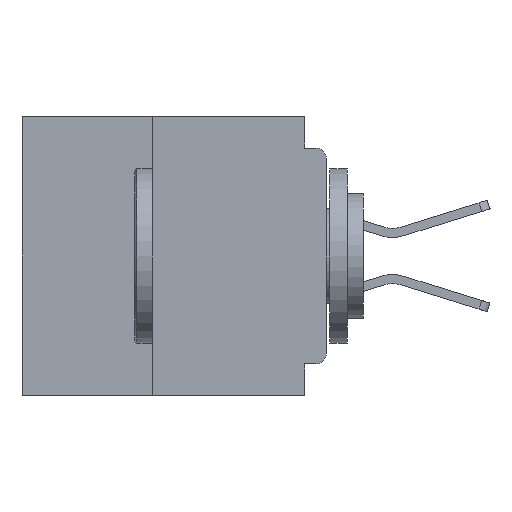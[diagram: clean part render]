
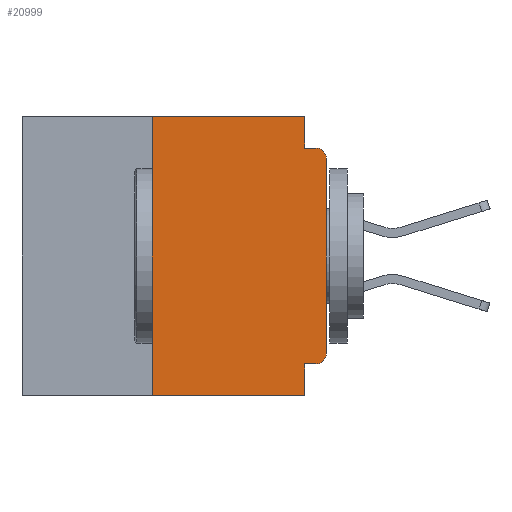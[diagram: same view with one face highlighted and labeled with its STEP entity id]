
A CAD part, left-side view. The second image highlights one B-rep face of the part: STEP entity #20999.
In plain terms, the highlighted planar face has unit normal (-1, 0, 0).
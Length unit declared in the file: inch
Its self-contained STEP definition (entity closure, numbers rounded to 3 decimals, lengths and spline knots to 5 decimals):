
#563 = EDGE_CURVE ( 'NONE', #13225, #25792, #38255, .T. ) ;
#1235 = DIRECTION ( 'NONE',  ( 0., -1., 0. ) ) ;
#1658 = CARTESIAN_POINT ( 'NONE',  ( 0., 0.031, -0.4 ) ) ;
#2220 = CARTESIAN_POINT ( 'NONE',  ( 0., 0.25, -0.4 ) ) ;
#3684 = CARTESIAN_POINT ( 'NONE',  ( 0., 0.015, -0.045 ) ) ;
#3929 = DIRECTION ( 'NONE',  ( 0., 1., 0. ) ) ;
#4262 = CARTESIAN_POINT ( 'NONE',  ( 0., 0., -0.06 ) ) ;
#4813 = LINE ( 'NONE', #6948, #27645 ) ;
#5031 = AXIS2_PLACEMENT_3D ( 'NONE', #33714, #15282, #36830 ) ;
#5234 = VECTOR ( 'NONE', #11529, 39.37008 ) ;
#6871 = CARTESIAN_POINT ( 'NONE',  ( 0., 0., 0. ) ) ;
#6878 = EDGE_CURVE ( 'NONE', #13225, #39548, #9457, .T. ) ;
#6948 = CARTESIAN_POINT ( 'NONE',  ( 0., 0., -0.355 ) ) ;
#8527 = DIRECTION ( 'NONE',  ( -1., 0., 0. ) ) ;
#9457 = LINE ( 'NONE', #17057, #16765 ) ;
#9583 = CARTESIAN_POINT ( 'NONE',  ( 0., 0.25, 0. ) ) ;
#9862 = CARTESIAN_POINT ( 'NONE',  ( 0., 0.031, -0.355 ) ) ;
#9892 = CARTESIAN_POINT ( 'NONE',  ( 0., 0.031, 0. ) ) ;
#10466 = CARTESIAN_POINT ( 'NONE',  ( 0., 0.437, 0. ) ) ;
#11529 = DIRECTION ( 'NONE',  ( 0., -1., 0. ) ) ;
#11684 = LINE ( 'NONE', #6871, #12640 ) ;
#11772 = EDGE_LOOP ( 'NONE', ( #24498, #18715, #12767, #12736, #38178, #14867, #18455, #31187, #39711, #34875 ) ) ;
#11964 = VERTEX_POINT ( 'NONE', #13065 ) ;
#12061 = CARTESIAN_POINT ( 'NONE',  ( 0., 0.437, -0.4 ) ) ;
#12195 = DIRECTION ( 'NONE',  ( 0., -1., 0. ) ) ;
#12214 = FACE_OUTER_BOUND ( 'NONE', #11772, .T. ) ;
#12640 = VECTOR ( 'NONE', #28558, 39.37008 ) ;
#12736 = ORIENTED_EDGE ( 'NONE', *, *, #13191, .F. ) ;
#12767 = ORIENTED_EDGE ( 'NONE', *, *, #37535, .F. ) ;
#13042 = VECTOR ( 'NONE', #1235, 39.37008 ) ;
#13065 = CARTESIAN_POINT ( 'NONE',  ( 0., 0.031, -0.045 ) ) ;
#13191 = EDGE_CURVE ( 'NONE', #37163, #11964, #19408, .T. ) ;
#13225 = VERTEX_POINT ( 'NONE', #2220 ) ;
#14592 = VECTOR ( 'NONE', #21707, 39.37008 ) ;
#14867 = ORIENTED_EDGE ( 'NONE', *, *, #6878, .F. ) ;
#15115 = AXIS2_PLACEMENT_3D ( 'NONE', #37827, #34837, #16387 ) ;
#15231 = AXIS2_PLACEMENT_3D ( 'NONE', #27081, #8527, #30190 ) ;
#15282 = DIRECTION ( 'NONE',  ( -1., 0., 0. ) ) ;
#15424 = CIRCLE ( 'NONE', #5031, 0.015 ) ;
#15717 = CARTESIAN_POINT ( 'NONE',  ( 0., 0.015, -0.355 ) ) ;
#16387 = DIRECTION ( 'NONE',  ( 0., 0., -1. ) ) ;
#16765 = VECTOR ( 'NONE', #26360, 39.37008 ) ;
#17057 = CARTESIAN_POINT ( 'NONE',  ( 0., 0.25, -0.4 ) ) ;
#18106 = VERTEX_POINT ( 'NONE', #4262 ) ;
#18455 = ORIENTED_EDGE ( 'NONE', *, *, #563, .T. ) ;
#18715 = ORIENTED_EDGE ( 'NONE', *, *, #38311, .T. ) ;
#19408 = LINE ( 'NONE', #29919, #34824 ) ;
#20945 = VERTEX_POINT ( 'NONE', #9862 ) ;
#20999 = ADVANCED_FACE ( 'NONE', ( #12214 ), #25551, .F. ) ;
#21025 = EDGE_CURVE ( 'NONE', #31451, #20945, #4813, .T. ) ;
#21286 = LINE ( 'NONE', #10466, #13042 ) ;
#21707 = DIRECTION ( 'NONE',  ( 0., 0., -1. ) ) ;
#22324 = EDGE_CURVE ( 'NONE', #34582, #18106, #11684, .T. ) ;
#22833 = LINE ( 'NONE', #37048, #14592 ) ;
#23974 = CARTESIAN_POINT ( 'NONE',  ( 0., 0., -0.045 ) ) ;
#24498 = ORIENTED_EDGE ( 'NONE', *, *, #22324, .T. ) ;
#25551 = PLANE ( 'NONE',  #15115 ) ;
#25792 = VERTEX_POINT ( 'NONE', #1658 ) ;
#25904 = EDGE_CURVE ( 'NONE', #31451, #34582, #27648, .T. ) ;
#26360 = DIRECTION ( 'NONE',  ( 0., 0., 1. ) ) ;
#26907 = VERTEX_POINT ( 'NONE', #3684 ) ;
#27081 = CARTESIAN_POINT ( 'NONE',  ( 0., 0.015, -0.34 ) ) ;
#27645 = VECTOR ( 'NONE', #3929, 39.37008 ) ;
#27648 = CIRCLE ( 'NONE', #15231, 0.015 ) ;
#28558 = DIRECTION ( 'NONE',  ( 0., 0., 1. ) ) ;
#29919 = CARTESIAN_POINT ( 'NONE',  ( 0., 0.031, 0. ) ) ;
#30190 = DIRECTION ( 'NONE',  ( 0., 0., -1. ) ) ;
#31187 = ORIENTED_EDGE ( 'NONE', *, *, #37014, .F. ) ;
#31451 = VERTEX_POINT ( 'NONE', #15717 ) ;
#31906 = LINE ( 'NONE', #23974, #5234 ) ;
#33714 = CARTESIAN_POINT ( 'NONE',  ( 0., 0.015, -0.06 ) ) ;
#34582 = VERTEX_POINT ( 'NONE', #36943 ) ;
#34824 = VECTOR ( 'NONE', #36109, 39.37008 ) ;
#34837 = DIRECTION ( 'NONE',  ( 1., 0., 0. ) ) ;
#34875 = ORIENTED_EDGE ( 'NONE', *, *, #25904, .T. ) ;
#34891 = EDGE_CURVE ( 'NONE', #39548, #37163, #21286, .T. ) ;
#36109 = DIRECTION ( 'NONE',  ( 0., 0., -1. ) ) ;
#36830 = DIRECTION ( 'NONE',  ( 0., 0., -1. ) ) ;
#36943 = CARTESIAN_POINT ( 'NONE',  ( 0., 0., -0.34 ) ) ;
#37014 = EDGE_CURVE ( 'NONE', #20945, #25792, #22833, .T. ) ;
#37048 = CARTESIAN_POINT ( 'NONE',  ( 0., 0.031, -0.4 ) ) ;
#37163 = VERTEX_POINT ( 'NONE', #9892 ) ;
#37277 = VECTOR ( 'NONE', #12195, 39.37008 ) ;
#37535 = EDGE_CURVE ( 'NONE', #11964, #26907, #31906, .T. ) ;
#37827 = CARTESIAN_POINT ( 'NONE',  ( 0., 0.437, 0. ) ) ;
#38178 = ORIENTED_EDGE ( 'NONE', *, *, #34891, .F. ) ;
#38255 = LINE ( 'NONE', #12061, #37277 ) ;
#38311 = EDGE_CURVE ( 'NONE', #18106, #26907, #15424, .T. ) ;
#39548 = VERTEX_POINT ( 'NONE', #9583 ) ;
#39711 = ORIENTED_EDGE ( 'NONE', *, *, #21025, .F. ) ;
